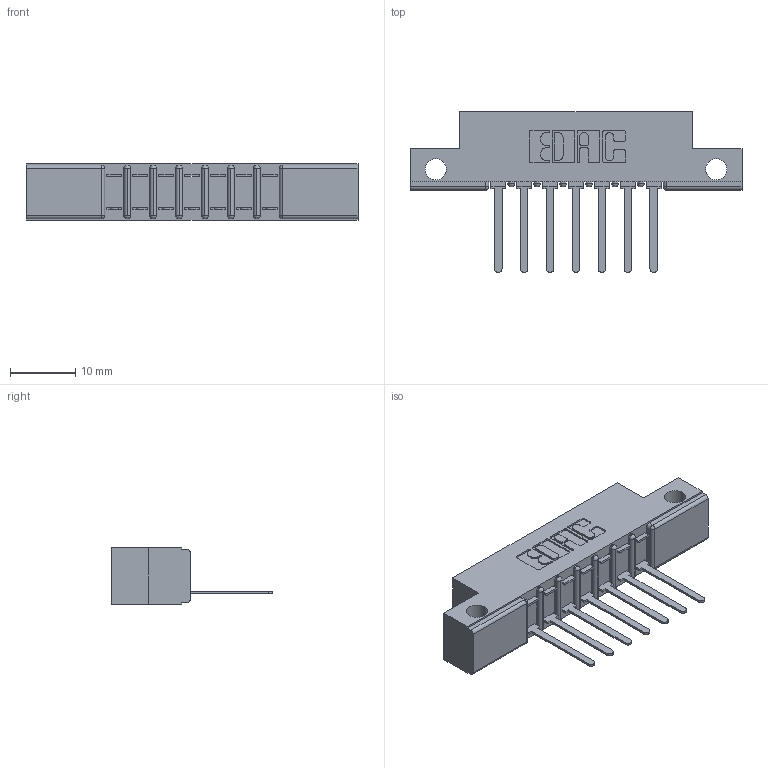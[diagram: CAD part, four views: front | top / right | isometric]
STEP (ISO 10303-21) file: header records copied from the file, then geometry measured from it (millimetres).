
FILE_DESCRIPTION (( 'STEP AP203' ), '1' );
FILE_NAME ('307-007-441-112.STEP', '2020-09-25T02:26:21', ( '' ), ( '' ), 'SwSTEP 2.0', 'SolidWorks 2020', '' );
FILE_SCHEMA (( 'CONFIG_CONTROL_DESIGN' ));
Length unit declared in the file: inch
Products named in the file (3): 307-290-002_541; 307-007-441-112; 307 Part_.128 Dia Side Mounting Holes
Assembly tree (8 placements, depth 2):
  307-007-441-112
    307 Part_.128 Dia Side Mounting Holes
    307-290-002_541  x7
Bounding box: 50.75 x 24.59 x 8.71 mm (x, y, z)
Volume: 3286.4 mm3; surface area: 5125 mm2
Topology: 8 solids, 8 shells, 644 faces, 1947 edges, 1274 vertices
Faces by surface type: plane 385, cylinder 243, sphere 16
Entity records: 11036 total; most frequent: CARTESIAN_POINT 1856, ORIENTED_EDGE 1846, DIRECTION 1819, EDGE_CURVE 923, LINE 689, VECTOR 689, VERTEX_POINT 602, AXIS2_PLACEMENT_3D 565
